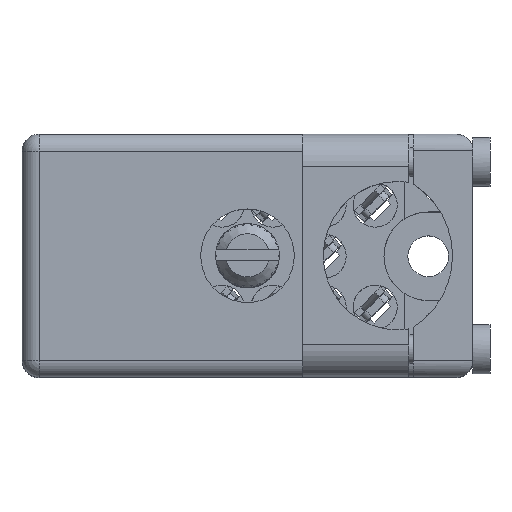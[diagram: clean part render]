
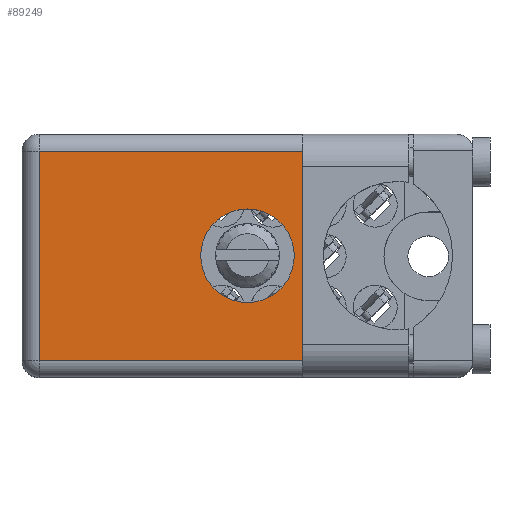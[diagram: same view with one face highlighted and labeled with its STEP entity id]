
A CAD part, top view. The second image highlights one B-rep face of the part: STEP entity #89249.
In plain terms, the highlighted face is planar.
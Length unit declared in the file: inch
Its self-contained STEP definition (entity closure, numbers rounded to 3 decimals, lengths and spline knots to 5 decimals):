
#1375 = ORIENTED_EDGE ( 'NONE', *, *, #19833, .T. ) ;
#2221 = LINE ( 'NONE', #120868, #46958 ) ;
#4560 = LINE ( 'NONE', #32268, #11156 ) ;
#8992 = VECTOR ( 'NONE', #109720, 39.37008 ) ;
#11156 = VECTOR ( 'NONE', #31013, 39.37008 ) ;
#11448 = DIRECTION ( 'NONE',  ( 0., 1., 0. ) ) ;
#13051 = VERTEX_POINT ( 'NONE', #134673 ) ;
#13889 = DIRECTION ( 'NONE',  ( 0., 0., 1. ) ) ;
#17307 = CARTESIAN_POINT ( 'NONE',  ( 0.05, 0.906, -0.665 ) ) ;
#17312 = CIRCLE ( 'NONE', #175184, 0.1375 ) ;
#19255 = DIRECTION ( 'NONE',  ( 1., 0., 0. ) ) ;
#19833 = EDGE_CURVE ( 'NONE', #123700, #78631, #159551, .T. ) ;
#23624 = CARTESIAN_POINT ( 'NONE',  ( 1.15, 0.906, -0.1125 ) ) ;
#24700 = EDGE_CURVE ( 'NONE', #151336, #123700, #4560, .T. ) ;
#26097 = EDGE_LOOP ( 'NONE', ( #160814, #27700 ) ) ;
#27700 = ORIENTED_EDGE ( 'NONE', *, *, #120421, .F. ) ;
#31013 = DIRECTION ( 'NONE',  ( -1., 0., 0. ) ) ;
#32268 = CARTESIAN_POINT ( 'NONE',  ( 0., 0.906, -0.665 ) ) ;
#38036 = DIRECTION ( 'NONE',  ( 0., 0., -1. ) ) ;
#39609 = ORIENTED_EDGE ( 'NONE', *, *, #105850, .T. ) ;
#39842 = CARTESIAN_POINT ( 'NONE',  ( 0.865, 0.906, -0.1125 ) ) ;
#41423 = VECTOR ( 'NONE', #19255, 39.37008 ) ;
#45426 = AXIS2_PLACEMENT_3D ( 'NONE', #70547, #157161, #156530 ) ;
#46958 = VECTOR ( 'NONE', #38036, 39.37008 ) ;
#48457 = DIRECTION ( 'NONE',  ( 0., 0., 1. ) ) ;
#57684 = CARTESIAN_POINT ( 'NONE',  ( 0.05, 0.906, -0.715 ) ) ;
#60496 = CARTESIAN_POINT ( 'NONE',  ( 0.05, 0.906, -0.05 ) ) ;
#66528 = VECTOR ( 'NONE', #146590, 39.37008 ) ;
#70547 = CARTESIAN_POINT ( 'NONE',  ( 0.6625, 0.906, -0.3575 ) ) ;
#72469 = ORIENTED_EDGE ( 'NONE', *, *, #84428, .F. ) ;
#73816 = DIRECTION ( 'NONE',  ( 0., 0., 1. ) ) ;
#75694 = CARTESIAN_POINT ( 'NONE',  ( 1.15, 0.906, -0.715 ) ) ;
#76519 = FACE_OUTER_BOUND ( 'NONE', #96106, .T. ) ;
#77033 = CARTESIAN_POINT ( 'NONE',  ( 1.15, 0.906, -0.05 ) ) ;
#78631 = VERTEX_POINT ( 'NONE', #60496 ) ;
#79511 = EDGE_CURVE ( 'NONE', #106484, #94426, #151920, .T. ) ;
#80140 = ORIENTED_EDGE ( 'NONE', *, *, #101548, .F. ) ;
#82727 = ORIENTED_EDGE ( 'NONE', *, *, #24700, .T. ) ;
#84428 = EDGE_CURVE ( 'NONE', #169803, #134732, #140047, .T. ) ;
#85504 = FACE_BOUND ( 'NONE', #26097, .T. ) ;
#89249 = ADVANCED_FACE ( 'NONE', ( #76519, #85504 ), #175031, .T. ) ;
#92486 = CARTESIAN_POINT ( 'NONE',  ( 1.15, 0.906, -0.05 ) ) ;
#94026 = CARTESIAN_POINT ( 'NONE',  ( 0.865, 0.906, -0.6025 ) ) ;
#94426 = VERTEX_POINT ( 'NONE', #177729 ) ;
#95298 = CARTESIAN_POINT ( 'NONE',  ( 0.865, 0.906, -0.1125 ) ) ;
#95415 = DIRECTION ( 'NONE',  ( 0., 1., 0. ) ) ;
#96106 = EDGE_LOOP ( 'NONE', ( #1375, #39609, #72469, #105043, #133738, #145001, #80140, #82727 ) ) ;
#98043 = CARTESIAN_POINT ( 'NONE',  ( 0.6625, 0.906, -0.22 ) ) ;
#99524 = VECTOR ( 'NONE', #48457, 39.37008 ) ;
#100626 = CARTESIAN_POINT ( 'NONE',  ( 1.15, 0.906, -0.715 ) ) ;
#101548 = EDGE_CURVE ( 'NONE', #151336, #94426, #169183, .T. ) ;
#103601 = VECTOR ( 'NONE', #112357, 39.37008 ) ;
#105043 = ORIENTED_EDGE ( 'NONE', *, *, #169602, .T. ) ;
#105850 = EDGE_CURVE ( 'NONE', #78631, #134732, #115563, .T. ) ;
#106484 = VERTEX_POINT ( 'NONE', #94026 ) ;
#109720 = DIRECTION ( 'NONE',  ( -1., 0., 0. ) ) ;
#110774 = VERTEX_POINT ( 'NONE', #98043 ) ;
#112357 = DIRECTION ( 'NONE',  ( 0., 0., 1. ) ) ;
#115563 = LINE ( 'NONE', #92486, #41423 ) ;
#117703 = CARTESIAN_POINT ( 'NONE',  ( 0.865, 0.906, -0.6025 ) ) ;
#119705 = EDGE_CURVE ( 'NONE', #110774, #13051, #17312, .T. ) ;
#119790 = VECTOR ( 'NONE', #73816, 39.37008 ) ;
#120421 = EDGE_CURVE ( 'NONE', #13051, #110774, #185360, .T. ) ;
#120868 = CARTESIAN_POINT ( 'NONE',  ( 0.865, 0.906, -0.1125 ) ) ;
#123700 = VERTEX_POINT ( 'NONE', #17307 ) ;
#129670 = EDGE_CURVE ( 'NONE', #170341, #106484, #2221, .T. ) ;
#133738 = ORIENTED_EDGE ( 'NONE', *, *, #129670, .T. ) ;
#134673 = CARTESIAN_POINT ( 'NONE',  ( 0.6625, 0.906, -0.495 ) ) ;
#134732 = VERTEX_POINT ( 'NONE', #77033 ) ;
#138093 = CARTESIAN_POINT ( 'NONE',  ( 0., 0.906, -0.715 ) ) ;
#140047 = LINE ( 'NONE', #100626, #99524 ) ;
#141268 = CARTESIAN_POINT ( 'NONE',  ( 0.6625, 0.906, -0.3575 ) ) ;
#145001 = ORIENTED_EDGE ( 'NONE', *, *, #79511, .T. ) ;
#146590 = DIRECTION ( 'NONE',  ( 1., 0., 0. ) ) ;
#151336 = VERTEX_POINT ( 'NONE', #169263 ) ;
#151920 = LINE ( 'NONE', #117703, #66528 ) ;
#154958 = LINE ( 'NONE', #95298, #8992 ) ;
#155070 = DIRECTION ( 'NONE',  ( 0., 0., 1. ) ) ;
#156530 = DIRECTION ( 'NONE',  ( 0., 0., 1. ) ) ;
#157161 = DIRECTION ( 'NONE',  ( 0., 1., 0. ) ) ;
#159551 = LINE ( 'NONE', #57684, #103601 ) ;
#160814 = ORIENTED_EDGE ( 'NONE', *, *, #119705, .F. ) ;
#164236 = AXIS2_PLACEMENT_3D ( 'NONE', #138093, #95415, #13889 ) ;
#169183 = LINE ( 'NONE', #75694, #119790 ) ;
#169263 = CARTESIAN_POINT ( 'NONE',  ( 1.15, 0.906, -0.665 ) ) ;
#169602 = EDGE_CURVE ( 'NONE', #169803, #170341, #154958, .T. ) ;
#169803 = VERTEX_POINT ( 'NONE', #23624 ) ;
#170341 = VERTEX_POINT ( 'NONE', #39842 ) ;
#175031 = PLANE ( 'NONE',  #164236 ) ;
#175184 = AXIS2_PLACEMENT_3D ( 'NONE', #141268, #11448, #155070 ) ;
#177729 = CARTESIAN_POINT ( 'NONE',  ( 1.15, 0.906, -0.6025 ) ) ;
#185360 = CIRCLE ( 'NONE', #45426, 0.1375 ) ;
